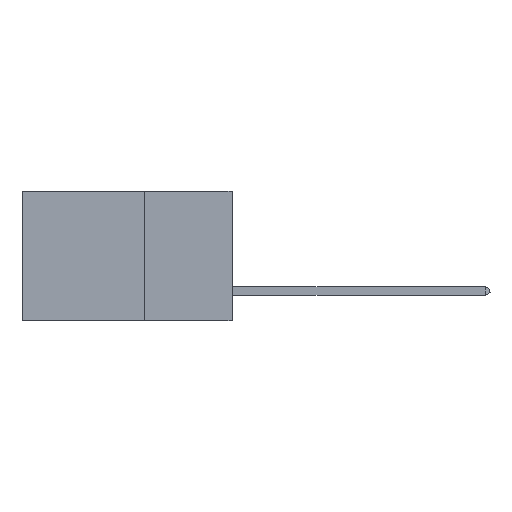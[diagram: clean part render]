
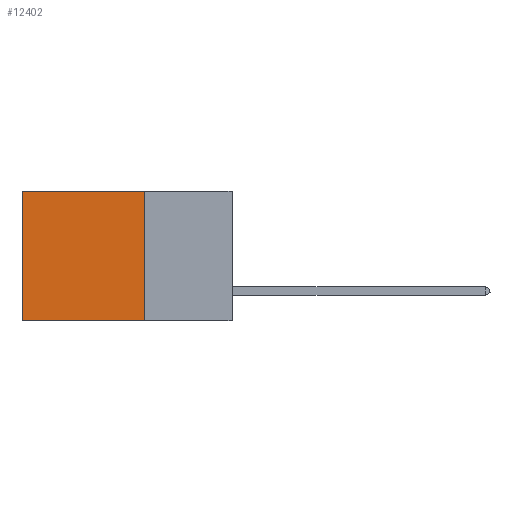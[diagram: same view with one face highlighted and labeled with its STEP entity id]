
A CAD part, left-side view. The second image highlights one B-rep face of the part: STEP entity #12402.
In plain terms, the highlighted planar face has unit normal (-1, 0, 0).
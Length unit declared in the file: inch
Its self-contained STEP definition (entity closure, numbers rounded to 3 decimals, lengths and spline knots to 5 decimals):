
#15 = CARTESIAN_POINT ( 'NONE',  ( 0.2875, 0.25, 0. ) ) ;
#4907 = EDGE_CURVE ( 'NONE', #7361, #11052, #8975, .T. ) ;
#5214 = VERTEX_POINT ( 'NONE', #16497 ) ;
#6337 = ORIENTED_EDGE ( 'NONE', *, *, #4907, .T. ) ;
#6557 = LINE ( 'NONE', #15, #12475 ) ;
#7016 = CARTESIAN_POINT ( 'NONE',  ( 0.2875, 0.25, 0. ) ) ;
#7059 = VECTOR ( 'NONE', #14984, 39.37008 ) ;
#7361 = VERTEX_POINT ( 'NONE', #22353 ) ;
#7614 = ORIENTED_EDGE ( 'NONE', *, *, #9339, .F. ) ;
#8586 = DIRECTION ( 'NONE',  ( 1., 0., 0. ) ) ;
#8975 = LINE ( 'NONE', #16693, #7059 ) ;
#9333 = LINE ( 'NONE', #20865, #15463 ) ;
#9339 = EDGE_CURVE ( 'NONE', #5214, #11052, #11949, .T. ) ;
#9855 = CARTESIAN_POINT ( 'NONE',  ( 0.2875, 0.6, -0.37 ) ) ;
#10398 = VECTOR ( 'NONE', #17829, 39.37008 ) ;
#10551 = FACE_OUTER_BOUND ( 'NONE', #11428, .T. ) ;
#11052 = VERTEX_POINT ( 'NONE', #9855 ) ;
#11428 = EDGE_LOOP ( 'NONE', ( #6337, #7614, #21668, #20996 ) ) ;
#11949 = LINE ( 'NONE', #12336, #10398 ) ;
#12336 = CARTESIAN_POINT ( 'NONE',  ( 0.2875, 0.25, -0.37 ) ) ;
#12402 = ADVANCED_FACE ( 'NONE', ( #10551 ), #16301, .F. ) ;
#12475 = VECTOR ( 'NONE', #23976, 39.37008 ) ;
#12766 = CARTESIAN_POINT ( 'NONE',  ( 0.2875, 0.25, 0. ) ) ;
#13438 = AXIS2_PLACEMENT_3D ( 'NONE', #12766, #8586, #16554 ) ;
#13858 = VERTEX_POINT ( 'NONE', #7016 ) ;
#14223 = EDGE_CURVE ( 'NONE', #13858, #5214, #9333, .T. ) ;
#14984 = DIRECTION ( 'NONE',  ( 0., 0., -1. ) ) ;
#15217 = DIRECTION ( 'NONE',  ( 0., 0., -1. ) ) ;
#15463 = VECTOR ( 'NONE', #15217, 39.37008 ) ;
#16301 = PLANE ( 'NONE',  #13438 ) ;
#16497 = CARTESIAN_POINT ( 'NONE',  ( 0.2875, 0.25, -0.37 ) ) ;
#16554 = DIRECTION ( 'NONE',  ( 0., 0., -1. ) ) ;
#16693 = CARTESIAN_POINT ( 'NONE',  ( 0.2875, 0.6, 0. ) ) ;
#17829 = DIRECTION ( 'NONE',  ( 0., 1., 0. ) ) ;
#19121 = EDGE_CURVE ( 'NONE', #13858, #7361, #6557, .T. ) ;
#20865 = CARTESIAN_POINT ( 'NONE',  ( 0.2875, 0.25, 0. ) ) ;
#20996 = ORIENTED_EDGE ( 'NONE', *, *, #19121, .T. ) ;
#21668 = ORIENTED_EDGE ( 'NONE', *, *, #14223, .F. ) ;
#22353 = CARTESIAN_POINT ( 'NONE',  ( 0.2875, 0.6, 0. ) ) ;
#23976 = DIRECTION ( 'NONE',  ( 0., 1., 0. ) ) ;
